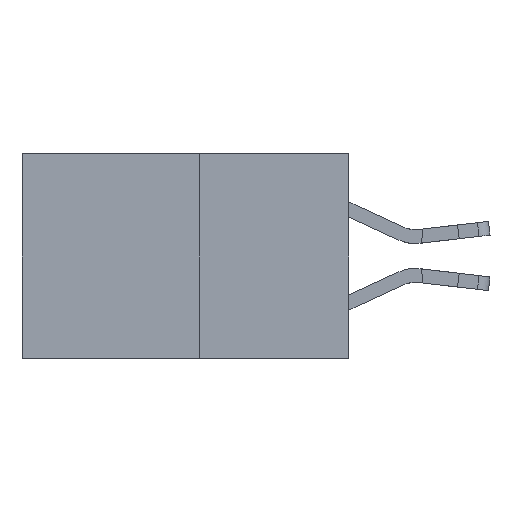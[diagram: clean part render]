
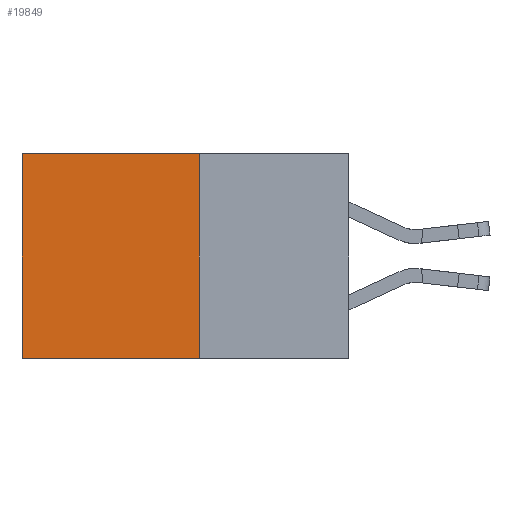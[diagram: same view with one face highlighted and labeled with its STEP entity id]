
A CAD part, left-side view. The second image highlights one B-rep face of the part: STEP entity #19849.
In plain terms, the highlighted planar face has unit normal (-1, 0, 0).
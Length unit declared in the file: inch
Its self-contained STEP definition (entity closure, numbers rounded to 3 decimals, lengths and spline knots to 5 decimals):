
#12 = EDGE_CURVE ( 'NONE', #18702, #15750, #15642, .T. ) ;
#818 = CARTESIAN_POINT ( 'NONE',  ( 0.277, 0.27, -0.37 ) ) ;
#1967 = VECTOR ( 'NONE', #6488, 39.37008 ) ;
#2528 = LINE ( 'NONE', #21503, #1967 ) ;
#4323 = ORIENTED_EDGE ( 'NONE', *, *, #19214, .T. ) ;
#4744 = CARTESIAN_POINT ( 'NONE',  ( 0.277, 0.59, 0. ) ) ;
#4783 = CARTESIAN_POINT ( 'NONE',  ( 0.277, 0.27, 0. ) ) ;
#6488 = DIRECTION ( 'NONE',  ( 0., 0., -1. ) ) ;
#7070 = VECTOR ( 'NONE', #13612, 39.37008 ) ;
#7712 = ORIENTED_EDGE ( 'NONE', *, *, #19877, .F. ) ;
#8206 = DIRECTION ( 'NONE',  ( 1., 0., 0. ) ) ;
#8503 = VERTEX_POINT ( 'NONE', #19040 ) ;
#8992 = AXIS2_PLACEMENT_3D ( 'NONE', #18278, #8206, #19921 ) ;
#9037 = LINE ( 'NONE', #9722, #21727 ) ;
#9722 = CARTESIAN_POINT ( 'NONE',  ( 0.277, 0.59, -0.37 ) ) ;
#11189 = VECTOR ( 'NONE', #19217, 39.37008 ) ;
#12346 = CARTESIAN_POINT ( 'NONE',  ( 0.277, 0.59, -0.37 ) ) ;
#13612 = DIRECTION ( 'NONE',  ( 0., 1., 0. ) ) ;
#15011 = PLANE ( 'NONE',  #8992 ) ;
#15642 = LINE ( 'NONE', #818, #11189 ) ;
#15750 = VERTEX_POINT ( 'NONE', #12346 ) ;
#16264 = VERTEX_POINT ( 'NONE', #4744 ) ;
#18126 = DIRECTION ( 'NONE',  ( 0., 0., -1. ) ) ;
#18278 = CARTESIAN_POINT ( 'NONE',  ( 0.277, 0.27, -0.37 ) ) ;
#18414 = ORIENTED_EDGE ( 'NONE', *, *, #18449, .T. ) ;
#18449 = EDGE_CURVE ( 'NONE', #16264, #15750, #9037, .T. ) ;
#18702 = VERTEX_POINT ( 'NONE', #18815 ) ;
#18815 = CARTESIAN_POINT ( 'NONE',  ( 0.277, 0.27, -0.37 ) ) ;
#19040 = CARTESIAN_POINT ( 'NONE',  ( 0.277, 0.27, 0. ) ) ;
#19214 = EDGE_CURVE ( 'NONE', #8503, #16264, #19955, .T. ) ;
#19217 = DIRECTION ( 'NONE',  ( 0., 1., 0. ) ) ;
#19849 = ADVANCED_FACE ( 'NONE', ( #20181 ), #15011, .F. ) ;
#19869 = EDGE_LOOP ( 'NONE', ( #18414, #20819, #7712, #4323 ) ) ;
#19877 = EDGE_CURVE ( 'NONE', #8503, #18702, #2528, .T. ) ;
#19921 = DIRECTION ( 'NONE',  ( 0., 0., -1. ) ) ;
#19955 = LINE ( 'NONE', #4783, #7070 ) ;
#20181 = FACE_OUTER_BOUND ( 'NONE', #19869, .T. ) ;
#20819 = ORIENTED_EDGE ( 'NONE', *, *, #12, .F. ) ;
#21503 = CARTESIAN_POINT ( 'NONE',  ( 0.277, 0.27, -0.37 ) ) ;
#21727 = VECTOR ( 'NONE', #18126, 39.37008 ) ;
